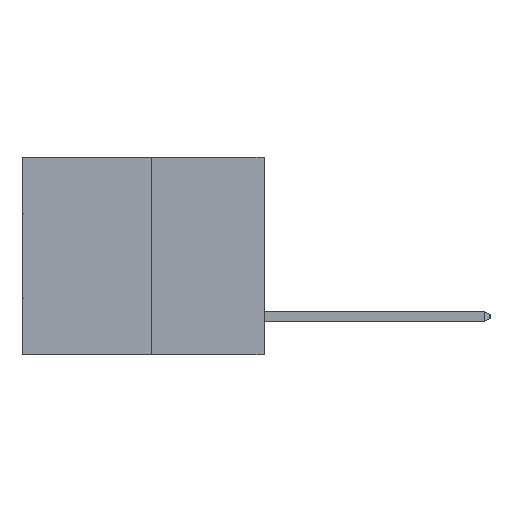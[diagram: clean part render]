
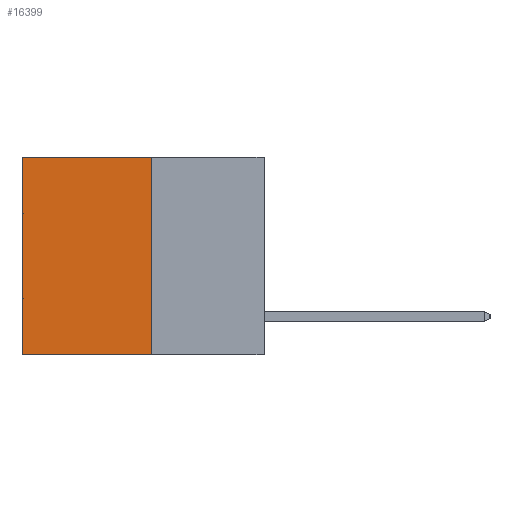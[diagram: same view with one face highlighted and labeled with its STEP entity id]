
A CAD part, left-side view. The second image highlights one B-rep face of the part: STEP entity #16399.
In plain terms, the highlighted planar face has unit normal (-1, 0, 0).
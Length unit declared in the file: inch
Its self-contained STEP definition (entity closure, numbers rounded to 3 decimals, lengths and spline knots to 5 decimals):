
#661 = FACE_OUTER_BOUND ( 'NONE', #28168, .T. ) ;
#1288 = VERTEX_POINT ( 'NONE', #9595 ) ;
#2075 = CARTESIAN_POINT ( 'NONE',  ( 0.3165, 0.28, 0. ) ) ;
#2568 = ORIENTED_EDGE ( 'NONE', *, *, #27366, .T. ) ;
#3076 = DIRECTION ( 'NONE',  ( 0., 1., 0. ) ) ;
#4612 = VERTEX_POINT ( 'NONE', #2075 ) ;
#4837 = VERTEX_POINT ( 'NONE', #17829 ) ;
#4933 = DIRECTION ( 'NONE',  ( 0., 1., 0. ) ) ;
#7216 = LINE ( 'NONE', #18810, #20282 ) ;
#9446 = DIRECTION ( 'NONE',  ( 0., 0., -1. ) ) ;
#9595 = CARTESIAN_POINT ( 'NONE',  ( 0.3165, 0.6, -0.49 ) ) ;
#10941 = EDGE_CURVE ( 'NONE', #4612, #23518, #14785, .T. ) ;
#12054 = CARTESIAN_POINT ( 'NONE',  ( 0.3165, 0.28, -0.49 ) ) ;
#12706 = VECTOR ( 'NONE', #3076, 39.37008 ) ;
#13178 = DIRECTION ( 'NONE',  ( 1., 0., 0. ) ) ;
#13379 = DIRECTION ( 'NONE',  ( 0., 0., -1. ) ) ;
#13667 = CARTESIAN_POINT ( 'NONE',  ( 0.3165, 0.6, -0.49 ) ) ;
#14061 = VECTOR ( 'NONE', #9446, 39.37008 ) ;
#14785 = LINE ( 'NONE', #29937, #14061 ) ;
#15839 = DIRECTION ( 'NONE',  ( 0., 0., -1. ) ) ;
#16399 = ADVANCED_FACE ( 'NONE', ( #661 ), #26950, .F. ) ;
#17713 = ORIENTED_EDGE ( 'NONE', *, *, #25685, .T. ) ;
#17829 = CARTESIAN_POINT ( 'NONE',  ( 0.3165, 0.6, 0. ) ) ;
#18234 = LINE ( 'NONE', #13667, #21852 ) ;
#18410 = ORIENTED_EDGE ( 'NONE', *, *, #26717, .F. ) ;
#18810 = CARTESIAN_POINT ( 'NONE',  ( 0.3165, 0.28, 0. ) ) ;
#19606 = LINE ( 'NONE', #29727, #12706 ) ;
#20282 = VECTOR ( 'NONE', #4933, 39.37008 ) ;
#20720 = ORIENTED_EDGE ( 'NONE', *, *, #10941, .F. ) ;
#21852 = VECTOR ( 'NONE', #15839, 39.37008 ) ;
#23518 = VERTEX_POINT ( 'NONE', #12054 ) ;
#25685 = EDGE_CURVE ( 'NONE', #4837, #1288, #18234, .T. ) ;
#26717 = EDGE_CURVE ( 'NONE', #23518, #1288, #19606, .T. ) ;
#26950 = PLANE ( 'NONE',  #29288 ) ;
#27047 = CARTESIAN_POINT ( 'NONE',  ( 0.3165, 0.28, -0.49 ) ) ;
#27366 = EDGE_CURVE ( 'NONE', #4612, #4837, #7216, .T. ) ;
#28168 = EDGE_LOOP ( 'NONE', ( #17713, #18410, #20720, #2568 ) ) ;
#29288 = AXIS2_PLACEMENT_3D ( 'NONE', #27047, #13178, #13379 ) ;
#29727 = CARTESIAN_POINT ( 'NONE',  ( 0.3165, 0.28, -0.49 ) ) ;
#29937 = CARTESIAN_POINT ( 'NONE',  ( 0.3165, 0.28, -0.49 ) ) ;
